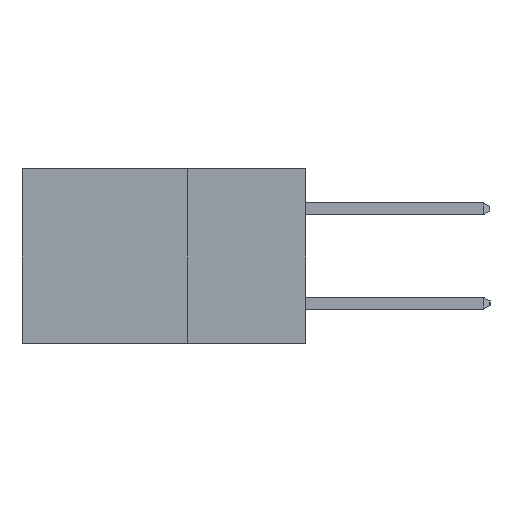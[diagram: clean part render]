
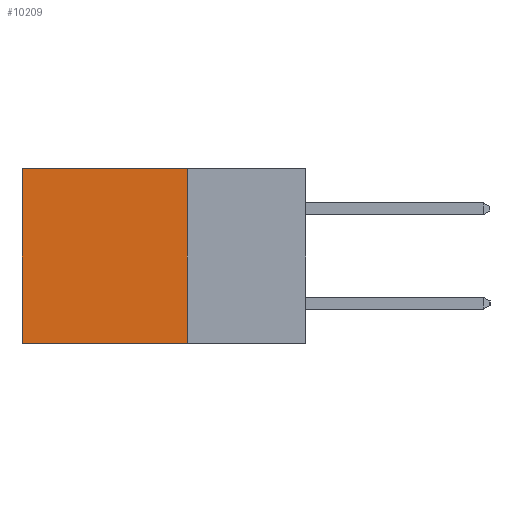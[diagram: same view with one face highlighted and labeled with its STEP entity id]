
A CAD part, left-side view. The second image highlights one B-rep face of the part: STEP entity #10209.
In plain terms, the highlighted planar face has unit normal (-1, 0, 0).
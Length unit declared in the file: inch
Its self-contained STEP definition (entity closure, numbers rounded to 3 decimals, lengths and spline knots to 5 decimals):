
#228 = CARTESIAN_POINT ( 'NONE',  ( 0.2615, 0.25, -0.37 ) ) ;
#1678 = EDGE_CURVE ( 'NONE', #6474, #7669, #2680, .T. ) ;
#2056 = LINE ( 'NONE', #3533, #9973 ) ;
#2680 = LINE ( 'NONE', #11123, #13147 ) ;
#2751 = ORIENTED_EDGE ( 'NONE', *, *, #11452, .T. ) ;
#2909 = DIRECTION ( 'NONE',  ( 0., 0., -1. ) ) ;
#2924 = CARTESIAN_POINT ( 'NONE',  ( 0.2615, 0.25, -0.37 ) ) ;
#2940 = DIRECTION ( 'NONE',  ( 1., 0., 0. ) ) ;
#2996 = DIRECTION ( 'NONE',  ( 0., 1., 0. ) ) ;
#3050 = PLANE ( 'NONE',  #7519 ) ;
#3063 = CARTESIAN_POINT ( 'NONE',  ( 0.2615, 0.25, -0.37 ) ) ;
#3466 = VERTEX_POINT ( 'NONE', #11060 ) ;
#3533 = CARTESIAN_POINT ( 'NONE',  ( 0.2615, 0.25, 0. ) ) ;
#4481 = CARTESIAN_POINT ( 'NONE',  ( 0.2615, 0.25, 0. ) ) ;
#5571 = DIRECTION ( 'NONE',  ( 0., 1., 0. ) ) ;
#6474 = VERTEX_POINT ( 'NONE', #4481 ) ;
#7158 = ORIENTED_EDGE ( 'NONE', *, *, #1678, .F. ) ;
#7348 = EDGE_LOOP ( 'NONE', ( #2751, #8482, #7158, #8723 ) ) ;
#7519 = AXIS2_PLACEMENT_3D ( 'NONE', #3063, #2940, #2909 ) ;
#7669 = VERTEX_POINT ( 'NONE', #2924 ) ;
#8482 = ORIENTED_EDGE ( 'NONE', *, *, #13300, .F. ) ;
#8680 = CARTESIAN_POINT ( 'NONE',  ( 0.2615, 0.6, 0. ) ) ;
#8723 = ORIENTED_EDGE ( 'NONE', *, *, #10807, .T. ) ;
#9195 = FACE_OUTER_BOUND ( 'NONE', #7348, .T. ) ;
#9278 = VERTEX_POINT ( 'NONE', #8680 ) ;
#9973 = VECTOR ( 'NONE', #2996, 39.37008 ) ;
#10209 = ADVANCED_FACE ( 'NONE', ( #9195 ), #3050, .F. ) ;
#10401 = VECTOR ( 'NONE', #5571, 39.37008 ) ;
#10431 = CARTESIAN_POINT ( 'NONE',  ( 0.2615, 0.6, -0.37 ) ) ;
#10628 = DIRECTION ( 'NONE',  ( 0., 0., -1. ) ) ;
#10807 = EDGE_CURVE ( 'NONE', #6474, #9278, #2056, .T. ) ;
#11060 = CARTESIAN_POINT ( 'NONE',  ( 0.2615, 0.6, -0.37 ) ) ;
#11123 = CARTESIAN_POINT ( 'NONE',  ( 0.2615, 0.25, -0.37 ) ) ;
#11452 = EDGE_CURVE ( 'NONE', #9278, #3466, #13205, .T. ) ;
#11634 = DIRECTION ( 'NONE',  ( 0., 0., -1. ) ) ;
#12591 = VECTOR ( 'NONE', #10628, 39.37008 ) ;
#13003 = LINE ( 'NONE', #228, #10401 ) ;
#13147 = VECTOR ( 'NONE', #11634, 39.37008 ) ;
#13205 = LINE ( 'NONE', #10431, #12591 ) ;
#13300 = EDGE_CURVE ( 'NONE', #7669, #3466, #13003, .T. ) ;
